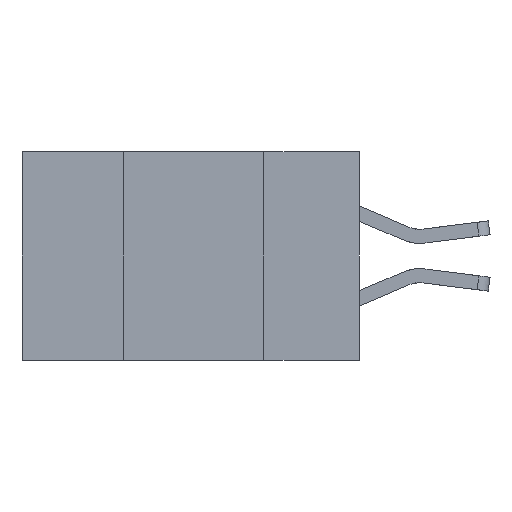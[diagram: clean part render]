
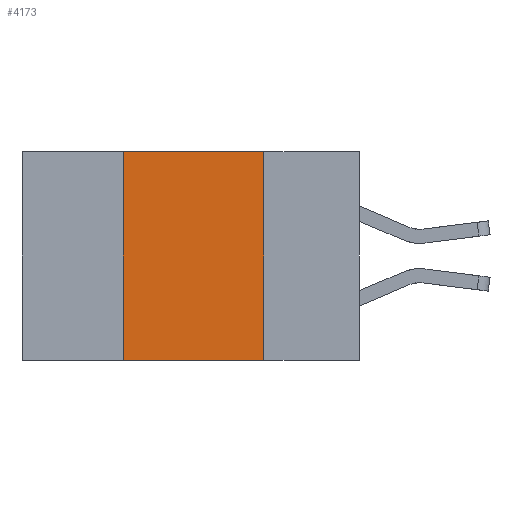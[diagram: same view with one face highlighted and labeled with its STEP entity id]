
A CAD part, left-side view. The second image highlights one B-rep face of the part: STEP entity #4173.
In plain terms, the highlighted planar face has unit normal (-1, 0, 0).
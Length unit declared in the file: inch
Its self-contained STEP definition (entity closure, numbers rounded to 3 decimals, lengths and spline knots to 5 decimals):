
#87 = EDGE_CURVE ( 'NONE', #5780, #7942, #7754, .T. ) ;
#522 = DIRECTION ( 'NONE',  ( 1., 0., 0. ) ) ;
#549 = LINE ( 'NONE', #1654, #7464 ) ;
#581 = VECTOR ( 'NONE', #9137, 39.37008 ) ;
#1527 = VECTOR ( 'NONE', #3035, 39.37008 ) ;
#1654 = CARTESIAN_POINT ( 'NONE',  ( 0., 0.17, 0. ) ) ;
#2278 = AXIS2_PLACEMENT_3D ( 'NONE', #5996, #522, #6856 ) ;
#2420 = PLANE ( 'NONE',  #2278 ) ;
#2431 = VERTEX_POINT ( 'NONE', #11029 ) ;
#3035 = DIRECTION ( 'NONE',  ( 0., -1., 0. ) ) ;
#3475 = DIRECTION ( 'NONE',  ( 0., 0., -1. ) ) ;
#4173 = ADVANCED_FACE ( 'NONE', ( #10037 ), #2420, .F. ) ;
#4694 = LINE ( 'NONE', #5270, #8963 ) ;
#5270 = CARTESIAN_POINT ( 'NONE',  ( 0., 0.42, 0. ) ) ;
#5340 = CARTESIAN_POINT ( 'NONE',  ( 0., 0.42, 0. ) ) ;
#5418 = CARTESIAN_POINT ( 'NONE',  ( 0., 0.42, -0.37 ) ) ;
#5780 = VERTEX_POINT ( 'NONE', #5340 ) ;
#5996 = CARTESIAN_POINT ( 'NONE',  ( 0., 0.6, 0. ) ) ;
#6366 = EDGE_CURVE ( 'NONE', #7942, #2431, #549, .T. ) ;
#6729 = CARTESIAN_POINT ( 'NONE',  ( 0., 0.17, 0. ) ) ;
#6856 = DIRECTION ( 'NONE',  ( 0., 0., -1. ) ) ;
#7367 = ORIENTED_EDGE ( 'NONE', *, *, #7535, .F. ) ;
#7464 = VECTOR ( 'NONE', #3475, 39.37008 ) ;
#7535 = EDGE_CURVE ( 'NONE', #11006, #5780, #4694, .T. ) ;
#7632 = ORIENTED_EDGE ( 'NONE', *, *, #10040, .T. ) ;
#7754 = LINE ( 'NONE', #9027, #581 ) ;
#7837 = DIRECTION ( 'NONE',  ( 0., 0., 1. ) ) ;
#7942 = VERTEX_POINT ( 'NONE', #6729 ) ;
#8550 = LINE ( 'NONE', #9098, #1527 ) ;
#8963 = VECTOR ( 'NONE', #7837, 39.37008 ) ;
#9026 = ORIENTED_EDGE ( 'NONE', *, *, #87, .F. ) ;
#9027 = CARTESIAN_POINT ( 'NONE',  ( 0., 0.6, 0. ) ) ;
#9098 = CARTESIAN_POINT ( 'NONE',  ( 0., 0.6, -0.37 ) ) ;
#9137 = DIRECTION ( 'NONE',  ( 0., -1., 0. ) ) ;
#9451 = EDGE_LOOP ( 'NONE', ( #10872, #9026, #7367, #7632 ) ) ;
#10037 = FACE_OUTER_BOUND ( 'NONE', #9451, .T. ) ;
#10040 = EDGE_CURVE ( 'NONE', #11006, #2431, #8550, .T. ) ;
#10872 = ORIENTED_EDGE ( 'NONE', *, *, #6366, .F. ) ;
#11006 = VERTEX_POINT ( 'NONE', #5418 ) ;
#11029 = CARTESIAN_POINT ( 'NONE',  ( 0., 0.17, -0.37 ) ) ;
